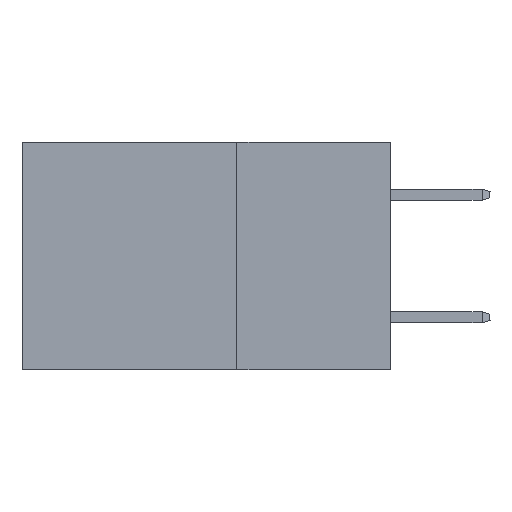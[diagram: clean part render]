
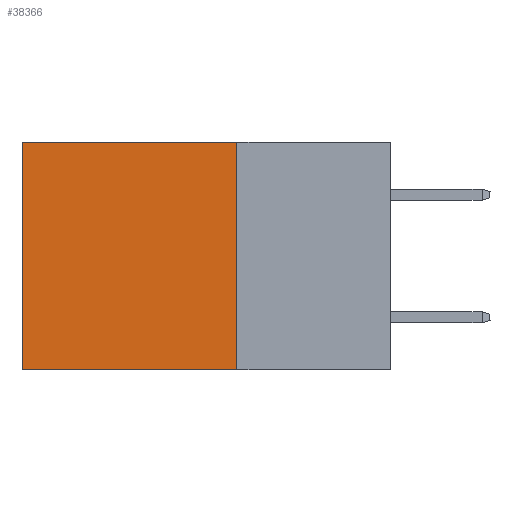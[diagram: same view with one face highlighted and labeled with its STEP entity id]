
A CAD part, left-side view. The second image highlights one B-rep face of the part: STEP entity #38366.
In plain terms, the highlighted planar face has unit normal (-1, 0, 0).
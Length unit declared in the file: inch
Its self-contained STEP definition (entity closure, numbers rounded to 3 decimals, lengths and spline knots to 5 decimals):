
#114 = LINE ( 'NONE', #31191, #16194 ) ;
#2784 = CARTESIAN_POINT ( 'NONE',  ( 0.2875, 0.25, 0. ) ) ;
#6990 = CARTESIAN_POINT ( 'NONE',  ( 0.2875, 0.6, -0.37 ) ) ;
#7305 = EDGE_CURVE ( 'NONE', #9986, #26765, #114, .T. ) ;
#7362 = ORIENTED_EDGE ( 'NONE', *, *, #27793, .T. ) ;
#9986 = VERTEX_POINT ( 'NONE', #39687 ) ;
#11137 = DIRECTION ( 'NONE',  ( 0., 1., 0. ) ) ;
#11204 = FACE_OUTER_BOUND ( 'NONE', #40863, .T. ) ;
#13714 = CARTESIAN_POINT ( 'NONE',  ( 0.2875, 0.25, 0. ) ) ;
#14788 = VECTOR ( 'NONE', #11137, 39.37008 ) ;
#15304 = EDGE_CURVE ( 'NONE', #9986, #41019, #29079, .T. ) ;
#16194 = VECTOR ( 'NONE', #27970, 39.37008 ) ;
#17090 = ORIENTED_EDGE ( 'NONE', *, *, #35832, .F. ) ;
#17212 = ORIENTED_EDGE ( 'NONE', *, *, #15304, .T. ) ;
#20132 = DIRECTION ( 'NONE',  ( 0., 0., -1. ) ) ;
#20307 = LINE ( 'NONE', #32770, #26729 ) ;
#23590 = PLANE ( 'NONE',  #28658 ) ;
#24549 = ORIENTED_EDGE ( 'NONE', *, *, #7305, .F. ) ;
#25264 = DIRECTION ( 'NONE',  ( 0., 1., 0. ) ) ;
#25920 = CARTESIAN_POINT ( 'NONE',  ( 0.2875, 0.6, 0. ) ) ;
#26729 = VECTOR ( 'NONE', #36124, 39.37008 ) ;
#26765 = VERTEX_POINT ( 'NONE', #33216 ) ;
#27793 = EDGE_CURVE ( 'NONE', #41019, #34347, #20307, .T. ) ;
#27970 = DIRECTION ( 'NONE',  ( 0., 0., -1. ) ) ;
#28658 = AXIS2_PLACEMENT_3D ( 'NONE', #13714, #36012, #20132 ) ;
#29079 = LINE ( 'NONE', #2784, #31564 ) ;
#31191 = CARTESIAN_POINT ( 'NONE',  ( 0.2875, 0.25, 0. ) ) ;
#31564 = VECTOR ( 'NONE', #25264, 39.37008 ) ;
#32770 = CARTESIAN_POINT ( 'NONE',  ( 0.2875, 0.6, 0. ) ) ;
#33216 = CARTESIAN_POINT ( 'NONE',  ( 0.2875, 0.25, -0.37 ) ) ;
#33430 = CARTESIAN_POINT ( 'NONE',  ( 0.2875, 0.25, -0.37 ) ) ;
#34347 = VERTEX_POINT ( 'NONE', #6990 ) ;
#35832 = EDGE_CURVE ( 'NONE', #26765, #34347, #36242, .T. ) ;
#36012 = DIRECTION ( 'NONE',  ( 1., 0., 0. ) ) ;
#36124 = DIRECTION ( 'NONE',  ( 0., 0., -1. ) ) ;
#36242 = LINE ( 'NONE', #33430, #14788 ) ;
#38366 = ADVANCED_FACE ( 'NONE', ( #11204 ), #23590, .F. ) ;
#39687 = CARTESIAN_POINT ( 'NONE',  ( 0.2875, 0.25, 0. ) ) ;
#40863 = EDGE_LOOP ( 'NONE', ( #7362, #17090, #24549, #17212 ) ) ;
#41019 = VERTEX_POINT ( 'NONE', #25920 ) ;
